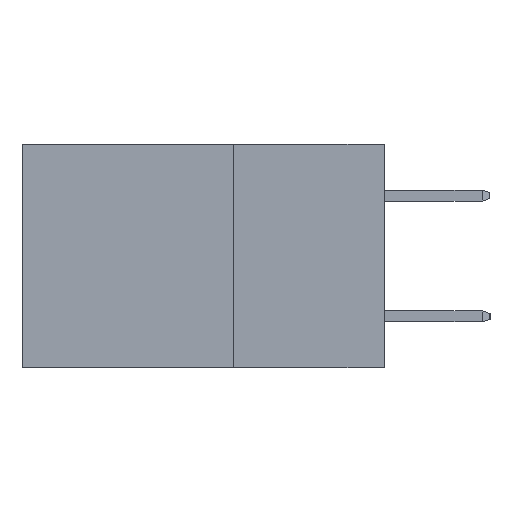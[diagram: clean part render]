
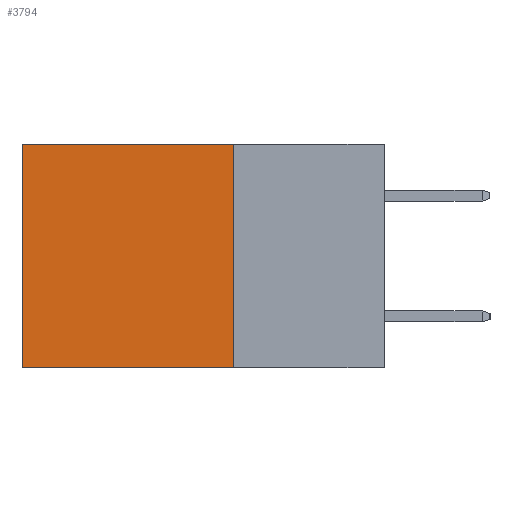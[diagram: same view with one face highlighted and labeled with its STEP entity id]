
A CAD part, left-side view. The second image highlights one B-rep face of the part: STEP entity #3794.
In plain terms, the highlighted planar face has unit normal (-1, 0, 0).
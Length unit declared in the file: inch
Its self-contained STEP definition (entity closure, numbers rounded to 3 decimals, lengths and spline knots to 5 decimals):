
#215 = PLANE ( 'NONE',  #9340 ) ;
#249 = CARTESIAN_POINT ( 'NONE',  ( 0.2615, 0.25, 0. ) ) ;
#371 = VECTOR ( 'NONE', #6997, 39.37008 ) ;
#592 = EDGE_CURVE ( 'NONE', #3898, #4680, #7832, .T. ) ;
#907 = VECTOR ( 'NONE', #6516, 39.37008 ) ;
#922 = VERTEX_POINT ( 'NONE', #6799 ) ;
#1737 = LINE ( 'NONE', #5422, #3417 ) ;
#1909 = CARTESIAN_POINT ( 'NONE',  ( 0.2615, 0.6, -0.37 ) ) ;
#2086 = EDGE_CURVE ( 'NONE', #6697, #3898, #6704, .T. ) ;
#2650 = VECTOR ( 'NONE', #3317, 39.37008 ) ;
#3163 = LINE ( 'NONE', #9225, #2650 ) ;
#3296 = FACE_OUTER_BOUND ( 'NONE', #5489, .T. ) ;
#3317 = DIRECTION ( 'NONE',  ( 0., 0., -1. ) ) ;
#3417 = VECTOR ( 'NONE', #6270, 39.37008 ) ;
#3794 = ADVANCED_FACE ( 'NONE', ( #3296 ), #215, .F. ) ;
#3898 = VERTEX_POINT ( 'NONE', #7616 ) ;
#3920 = ORIENTED_EDGE ( 'NONE', *, *, #4088, .F. ) ;
#4088 = EDGE_CURVE ( 'NONE', #6697, #922, #3163, .T. ) ;
#4149 = ORIENTED_EDGE ( 'NONE', *, *, #2086, .T. ) ;
#4680 = VERTEX_POINT ( 'NONE', #1909 ) ;
#5422 = CARTESIAN_POINT ( 'NONE',  ( 0.2615, 0.25, -0.37 ) ) ;
#5489 = EDGE_LOOP ( 'NONE', ( #7622, #6593, #3920, #4149 ) ) ;
#6270 = DIRECTION ( 'NONE',  ( 0., 1., 0. ) ) ;
#6516 = DIRECTION ( 'NONE',  ( 0., 0., -1. ) ) ;
#6593 = ORIENTED_EDGE ( 'NONE', *, *, #8926, .F. ) ;
#6622 = CARTESIAN_POINT ( 'NONE',  ( 0.2615, 0.6, -0.37 ) ) ;
#6697 = VERTEX_POINT ( 'NONE', #249 ) ;
#6704 = LINE ( 'NONE', #6969, #371 ) ;
#6799 = CARTESIAN_POINT ( 'NONE',  ( 0.2615, 0.25, -0.37 ) ) ;
#6969 = CARTESIAN_POINT ( 'NONE',  ( 0.2615, 0.25, 0. ) ) ;
#6997 = DIRECTION ( 'NONE',  ( 0., 1., 0. ) ) ;
#7616 = CARTESIAN_POINT ( 'NONE',  ( 0.2615, 0.6, 0. ) ) ;
#7622 = ORIENTED_EDGE ( 'NONE', *, *, #592, .T. ) ;
#7832 = LINE ( 'NONE', #6622, #907 ) ;
#8926 = EDGE_CURVE ( 'NONE', #922, #4680, #1737, .T. ) ;
#9225 = CARTESIAN_POINT ( 'NONE',  ( 0.2615, 0.25, -0.37 ) ) ;
#9340 = AXIS2_PLACEMENT_3D ( 'NONE', #10735, #10636, #10613 ) ;
#10613 = DIRECTION ( 'NONE',  ( 0., 0., -1. ) ) ;
#10636 = DIRECTION ( 'NONE',  ( 1., 0., 0. ) ) ;
#10735 = CARTESIAN_POINT ( 'NONE',  ( 0.2615, 0.25, -0.37 ) ) ;
